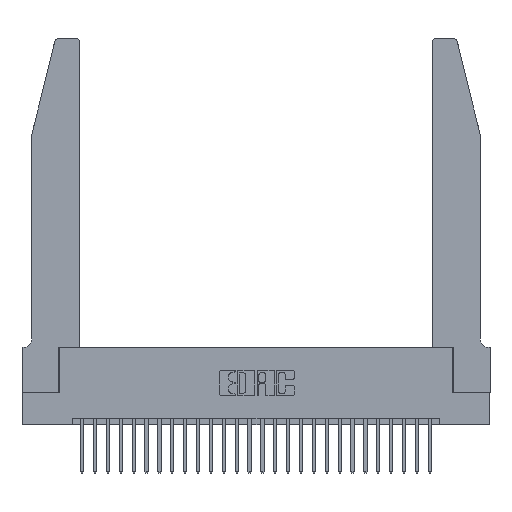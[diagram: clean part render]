
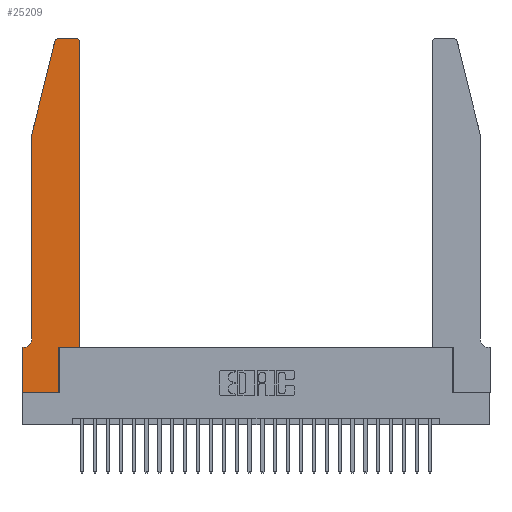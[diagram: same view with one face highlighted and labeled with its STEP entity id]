
A CAD part, top view. The second image highlights one B-rep face of the part: STEP entity #25209.
In plain terms, the highlighted planar face has unit normal (0, 0, 1).
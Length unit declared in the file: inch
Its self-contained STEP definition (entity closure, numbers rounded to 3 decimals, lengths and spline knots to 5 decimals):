
#83 = ORIENTED_EDGE ( 'NONE', *, *, #17797, .T. ) ;
#126 = ORIENTED_EDGE ( 'NONE', *, *, #6767, .T. ) ;
#255 = CARTESIAN_POINT ( 'NONE',  ( 0.0755, 0.42, 0.37 ) ) ;
#271 = VECTOR ( 'NONE', #8926, 39.37008 ) ;
#326 = VECTOR ( 'NONE', #22467, 39.37008 ) ;
#510 = VERTEX_POINT ( 'NONE', #22723 ) ;
#595 = CIRCLE ( 'NONE', #19276, 0.03 ) ;
#699 = ORIENTED_EDGE ( 'NONE', *, *, #7916, .T. ) ;
#1030 = LINE ( 'NONE', #20239, #326 ) ;
#1064 = VERTEX_POINT ( 'NONE', #16920 ) ;
#1346 = LINE ( 'NONE', #27736, #24187 ) ;
#1620 = ORIENTED_EDGE ( 'NONE', *, *, #7390, .T. ) ;
#1651 = LINE ( 'NONE', #19138, #6861 ) ;
#1832 = DIRECTION ( 'NONE',  ( -1., 0., 0. ) ) ;
#2013 = LINE ( 'NONE', #23890, #25540 ) ;
#2141 = CARTESIAN_POINT ( 'NONE',  ( 0.2865, 0.35, 0.37 ) ) ;
#2415 = VERTEX_POINT ( 'NONE', #25924 ) ;
#2540 = CARTESIAN_POINT ( 'NONE',  ( 0.2865, 0., 0.37 ) ) ;
#2930 = ORIENTED_EDGE ( 'NONE', *, *, #20167, .T. ) ;
#2956 = VECTOR ( 'NONE', #6271, 39.37008 ) ;
#3343 = VERTEX_POINT ( 'NONE', #8903 ) ;
#3424 = EDGE_CURVE ( 'NONE', #16320, #12005, #6036, .T. ) ;
#3662 = DIRECTION ( 'NONE',  ( 0., -1., 0. ) ) ;
#4033 = CARTESIAN_POINT ( 'NONE',  ( 0., 0., 0.37 ) ) ;
#4424 = ORIENTED_EDGE ( 'NONE', *, *, #14918, .T. ) ;
#4798 = ORIENTED_EDGE ( 'NONE', *, *, #23047, .T. ) ;
#5124 = ORIENTED_EDGE ( 'NONE', *, *, #21179, .T. ) ;
#5450 = VERTEX_POINT ( 'NONE', #27752 ) ;
#6036 = LINE ( 'NONE', #24617, #17785 ) ;
#6262 = DIRECTION ( 'NONE',  ( 0., 0., -1. ) ) ;
#6271 = DIRECTION ( 'NONE',  ( 1., 0., 0. ) ) ;
#6652 = CARTESIAN_POINT ( 'NONE',  ( 0.4205, 2.72, 0.37 ) ) ;
#6757 = CARTESIAN_POINT ( 'NONE',  ( 0., 0.35, 0.37 ) ) ;
#6767 = EDGE_CURVE ( 'NONE', #21221, #16320, #16631, .T. ) ;
#6861 = VECTOR ( 'NONE', #3662, 39.37008 ) ;
#6888 = CARTESIAN_POINT ( 'NONE',  ( 0.0055, 0.35, 0.37 ) ) ;
#7390 = EDGE_CURVE ( 'NONE', #3343, #5450, #2013, .T. ) ;
#7916 = EDGE_CURVE ( 'NONE', #23982, #3343, #595, .T. ) ;
#8894 = DIRECTION ( 'NONE',  ( 1., 0., 0. ) ) ;
#8903 = CARTESIAN_POINT ( 'NONE',  ( 0.4205, 2.75, 0.37 ) ) ;
#8926 = DIRECTION ( 'NONE',  ( -0.239, -0.971, 0. ) ) ;
#8998 = DIRECTION ( 'NONE',  ( 0., 0., 1. ) ) ;
#10599 = ORIENTED_EDGE ( 'NONE', *, *, #21621, .T. ) ;
#10747 = CARTESIAN_POINT ( 'NONE',  ( 0., 0.35, 0.37 ) ) ;
#11405 = LINE ( 'NONE', #24360, #271 ) ;
#12005 = VERTEX_POINT ( 'NONE', #10747 ) ;
#12487 = CARTESIAN_POINT ( 'NONE',  ( 0.284, 2.72, 0.37 ) ) ;
#13437 = VERTEX_POINT ( 'NONE', #2141 ) ;
#13472 = ORIENTED_EDGE ( 'NONE', *, *, #20905, .T. ) ;
#14536 = EDGE_CURVE ( 'NONE', #5450, #510, #21112, .T. ) ;
#14699 = DIRECTION ( 'NONE',  ( 1., 0., 0. ) ) ;
#14907 = VERTEX_POINT ( 'NONE', #2540 ) ;
#14918 = EDGE_CURVE ( 'NONE', #14907, #13437, #1030, .T. ) ;
#16320 = VERTEX_POINT ( 'NONE', #6888 ) ;
#16523 = DIRECTION ( 'NONE',  ( 1., 0., 0. ) ) ;
#16631 = CIRCLE ( 'NONE', #21780, 0.07 ) ;
#16754 = VECTOR ( 'NONE', #18694, 39.37008 ) ;
#16776 = DIRECTION ( 'NONE',  ( 0., -1., 0. ) ) ;
#16920 = CARTESIAN_POINT ( 'NONE',  ( 0., 0., 0.37 ) ) ;
#17785 = VECTOR ( 'NONE', #26718, 39.37008 ) ;
#17797 = EDGE_CURVE ( 'NONE', #2415, #23982, #22592, .T. ) ;
#18591 = CARTESIAN_POINT ( 'NONE',  ( 0.4505, 2.72, 0.37 ) ) ;
#18694 = DIRECTION ( 'NONE',  ( 0., 1., 0. ) ) ;
#18770 = FACE_OUTER_BOUND ( 'NONE', #22739, .T. ) ;
#19138 = CARTESIAN_POINT ( 'NONE',  ( 0.0755, 2., 0.37 ) ) ;
#19276 = AXIS2_PLACEMENT_3D ( 'NONE', #6652, #22093, #8894 ) ;
#19497 = CARTESIAN_POINT ( 'NONE',  ( 0.0055, 0.42, 0.37 ) ) ;
#19992 = PLANE ( 'NONE',  #28211 ) ;
#20167 = EDGE_CURVE ( 'NONE', #13437, #2415, #26621, .T. ) ;
#20234 = VERTEX_POINT ( 'NONE', #23440 ) ;
#20239 = CARTESIAN_POINT ( 'NONE',  ( 0.2865, 0.35, 0.37 ) ) ;
#20600 = LINE ( 'NONE', #4033, #2956 ) ;
#20760 = VECTOR ( 'NONE', #16523, 39.37008 ) ;
#20905 = EDGE_CURVE ( 'NONE', #12005, #1064, #1346, .T. ) ;
#21112 = CIRCLE ( 'NONE', #23622, 0.03 ) ;
#21179 = EDGE_CURVE ( 'NONE', #510, #20234, #11405, .T. ) ;
#21221 = VERTEX_POINT ( 'NONE', #255 ) ;
#21621 = EDGE_CURVE ( 'NONE', #20234, #21221, #1651, .T. ) ;
#21698 = DIRECTION ( 'NONE',  ( -1., 0., 0. ) ) ;
#21780 = AXIS2_PLACEMENT_3D ( 'NONE', #19497, #6262, #21698 ) ;
#21899 = ORIENTED_EDGE ( 'NONE', *, *, #3424, .T. ) ;
#22093 = DIRECTION ( 'NONE',  ( 0., 0., 1. ) ) ;
#22467 = DIRECTION ( 'NONE',  ( 0., 1., 0. ) ) ;
#22592 = LINE ( 'NONE', #25264, #16754 ) ;
#22723 = CARTESIAN_POINT ( 'NONE',  ( 0.25487, 2.72718, 0.37 ) ) ;
#22739 = EDGE_LOOP ( 'NONE', ( #1620, #24757, #5124, #10599, #126, #21899, #13472, #4798, #4424, #2930, #83, #699 ) ) ;
#23047 = EDGE_CURVE ( 'NONE', #1064, #14907, #20600, .T. ) ;
#23440 = CARTESIAN_POINT ( 'NONE',  ( 0.0755, 2., 0.37 ) ) ;
#23622 = AXIS2_PLACEMENT_3D ( 'NONE', #12487, #27886, #14699 ) ;
#23890 = CARTESIAN_POINT ( 'NONE',  ( 0.2605, 2.75, 0.37 ) ) ;
#23982 = VERTEX_POINT ( 'NONE', #18591 ) ;
#24187 = VECTOR ( 'NONE', #16776, 39.37008 ) ;
#24360 = CARTESIAN_POINT ( 'NONE',  ( 0.0755, 2., 0.37 ) ) ;
#24424 = DIRECTION ( 'NONE',  ( 1., 0., 0. ) ) ;
#24617 = CARTESIAN_POINT ( 'NONE',  ( 0.0755, 0.35, 0.37 ) ) ;
#24757 = ORIENTED_EDGE ( 'NONE', *, *, #14536, .T. ) ;
#25209 = ADVANCED_FACE ( 'NONE', ( #18770 ), #19992, .T. ) ;
#25264 = CARTESIAN_POINT ( 'NONE',  ( 0.4505, 0.35, 0.37 ) ) ;
#25374 = CARTESIAN_POINT ( 'NONE',  ( 0.4505, 0.35, 0.37 ) ) ;
#25540 = VECTOR ( 'NONE', #1832, 39.37008 ) ;
#25924 = CARTESIAN_POINT ( 'NONE',  ( 0.4505, 0.35, 0.37 ) ) ;
#26621 = LINE ( 'NONE', #25374, #20760 ) ;
#26718 = DIRECTION ( 'NONE',  ( -1., 0., 0. ) ) ;
#27736 = CARTESIAN_POINT ( 'NONE',  ( 0., 0., 0.37 ) ) ;
#27752 = CARTESIAN_POINT ( 'NONE',  ( 0.284, 2.75, 0.37 ) ) ;
#27886 = DIRECTION ( 'NONE',  ( 0., 0., 1. ) ) ;
#28211 = AXIS2_PLACEMENT_3D ( 'NONE', #6757, #8998, #24424 ) ;
